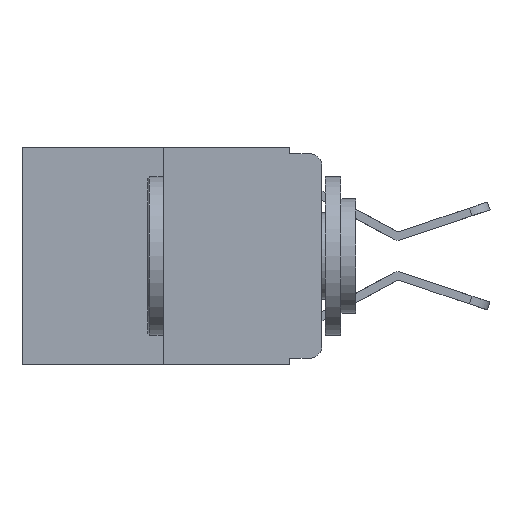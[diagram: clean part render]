
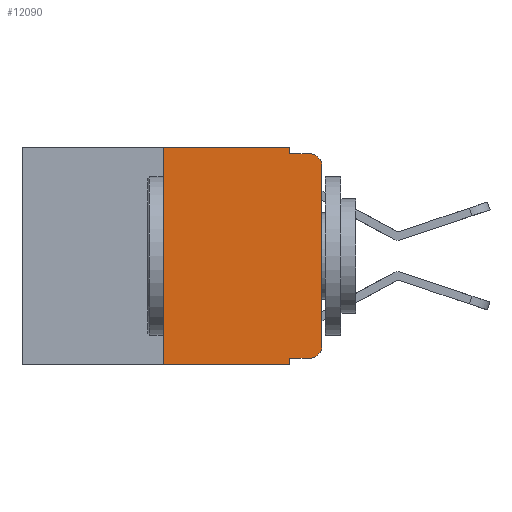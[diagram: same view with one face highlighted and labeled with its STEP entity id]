
A CAD part, left-side view. The second image highlights one B-rep face of the part: STEP entity #12090.
In plain terms, the highlighted planar face has unit normal (-1, 0, 0).
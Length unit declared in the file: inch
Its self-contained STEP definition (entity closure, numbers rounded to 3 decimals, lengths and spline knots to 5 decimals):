
#11 = VECTOR ( 'NONE', #6923, 39.37008 ) ;
#379 = LINE ( 'NONE', #5913, #11 ) ;
#500 = VERTEX_POINT ( 'NONE', #4023 ) ;
#547 = CARTESIAN_POINT ( 'NONE',  ( 0., 0.25, -0.343 ) ) ;
#619 = EDGE_CURVE ( 'NONE', #12169, #500, #5837, .T. ) ;
#708 = CARTESIAN_POINT ( 'NONE',  ( 0., 0.473, -0.343 ) ) ;
#769 = VECTOR ( 'NONE', #8160, 39.37008 ) ;
#1096 = ORIENTED_EDGE ( 'NONE', *, *, #5232, .T. ) ;
#1270 = VECTOR ( 'NONE', #1719, 39.37008 ) ;
#1434 = CARTESIAN_POINT ( 'NONE',  ( 0., 0.051, -0.343 ) ) ;
#1558 = AXIS2_PLACEMENT_3D ( 'NONE', #4679, #11574, #5676 ) ;
#1619 = LINE ( 'NONE', #3967, #1270 ) ;
#1627 = DIRECTION ( 'NONE',  ( 0., 0., -1. ) ) ;
#1719 = DIRECTION ( 'NONE',  ( 0., 0., 1. ) ) ;
#1965 = VERTEX_POINT ( 'NONE', #9014 ) ;
#2000 = ORIENTED_EDGE ( 'NONE', *, *, #619, .F. ) ;
#2155 = AXIS2_PLACEMENT_3D ( 'NONE', #3371, #3324, #12290 ) ;
#2701 = ORIENTED_EDGE ( 'NONE', *, *, #8767, .T. ) ;
#2798 = VECTOR ( 'NONE', #7585, 39.37008 ) ;
#2803 = VERTEX_POINT ( 'NONE', #3824 ) ;
#3264 = EDGE_LOOP ( 'NONE', ( #10030, #10320, #11503, #3905, #2000, #12675, #2701, #10756, #1096, #9434 ) ) ;
#3324 = DIRECTION ( 'NONE',  ( 1., 0., 0. ) ) ;
#3371 = CARTESIAN_POINT ( 'NONE',  ( 0., 0.473, 0. ) ) ;
#3824 = CARTESIAN_POINT ( 'NONE',  ( 0., 0.051, -0.01 ) ) ;
#3861 = EDGE_CURVE ( 'NONE', #9322, #11887, #9301, .T. ) ;
#3905 = ORIENTED_EDGE ( 'NONE', *, *, #7930, .F. ) ;
#3967 = CARTESIAN_POINT ( 'NONE',  ( 0., 0., 0. ) ) ;
#4023 = CARTESIAN_POINT ( 'NONE',  ( 0., 0.051, 0. ) ) ;
#4426 = DIRECTION ( 'NONE',  ( 0., 0., 1. ) ) ;
#4561 = DIRECTION ( 'NONE',  ( 0., -1., 0. ) ) ;
#4667 = CARTESIAN_POINT ( 'NONE',  ( 0., 0.051, -0.333 ) ) ;
#4679 = CARTESIAN_POINT ( 'NONE',  ( 0., 0.02, -0.03 ) ) ;
#5080 = CARTESIAN_POINT ( 'NONE',  ( 0., 0., -0.313 ) ) ;
#5232 = EDGE_CURVE ( 'NONE', #1965, #9322, #8145, .T. ) ;
#5574 = LINE ( 'NONE', #10499, #2798 ) ;
#5676 = DIRECTION ( 'NONE',  ( 0., 0., -1. ) ) ;
#5837 = LINE ( 'NONE', #6064, #10786 ) ;
#5873 = CARTESIAN_POINT ( 'NONE',  ( 0., 0.051, 0. ) ) ;
#5888 = EDGE_CURVE ( 'NONE', #1965, #7457, #10716, .T. ) ;
#5913 = CARTESIAN_POINT ( 'NONE',  ( 0., 0.051, -0.01 ) ) ;
#6064 = CARTESIAN_POINT ( 'NONE',  ( 0., 0.473, 0. ) ) ;
#6923 = DIRECTION ( 'NONE',  ( 0., -1., 0. ) ) ;
#6982 = VERTEX_POINT ( 'NONE', #547 ) ;
#7156 = LINE ( 'NONE', #10394, #12323 ) ;
#7219 = CARTESIAN_POINT ( 'NONE',  ( 0., 0., -0.03 ) ) ;
#7250 = EDGE_CURVE ( 'NONE', #6982, #12169, #7156, .T. ) ;
#7457 = VERTEX_POINT ( 'NONE', #1434 ) ;
#7585 = DIRECTION ( 'NONE',  ( 0., 0., -1. ) ) ;
#7930 = EDGE_CURVE ( 'NONE', #500, #2803, #5574, .T. ) ;
#8145 = LINE ( 'NONE', #4667, #13220 ) ;
#8150 = VECTOR ( 'NONE', #1627, 39.37008 ) ;
#8160 = DIRECTION ( 'NONE',  ( 0., -1., 0. ) ) ;
#8767 = EDGE_CURVE ( 'NONE', #6982, #7457, #11999, .T. ) ;
#9014 = CARTESIAN_POINT ( 'NONE',  ( 0., 0.051, -0.333 ) ) ;
#9268 = EDGE_CURVE ( 'NONE', #2803, #11453, #379, .T. ) ;
#9301 = CIRCLE ( 'NONE', #9639, 0.02 ) ;
#9322 = VERTEX_POINT ( 'NONE', #10923 ) ;
#9434 = ORIENTED_EDGE ( 'NONE', *, *, #3861, .T. ) ;
#9639 = AXIS2_PLACEMENT_3D ( 'NONE', #9780, #10190, #10152 ) ;
#9780 = CARTESIAN_POINT ( 'NONE',  ( 0., 0.02, -0.313 ) ) ;
#9903 = CIRCLE ( 'NONE', #1558, 0.02 ) ;
#10030 = ORIENTED_EDGE ( 'NONE', *, *, #11810, .T. ) ;
#10152 = DIRECTION ( 'NONE',  ( 0., 0., -1. ) ) ;
#10190 = DIRECTION ( 'NONE',  ( -1., 0., 0. ) ) ;
#10320 = ORIENTED_EDGE ( 'NONE', *, *, #10549, .T. ) ;
#10394 = CARTESIAN_POINT ( 'NONE',  ( 0., 0.25, 0. ) ) ;
#10499 = CARTESIAN_POINT ( 'NONE',  ( 0., 0.051, 0. ) ) ;
#10549 = EDGE_CURVE ( 'NONE', #10863, #11453, #9903, .T. ) ;
#10716 = LINE ( 'NONE', #5873, #8150 ) ;
#10756 = ORIENTED_EDGE ( 'NONE', *, *, #5888, .F. ) ;
#10786 = VECTOR ( 'NONE', #11528, 39.37008 ) ;
#10863 = VERTEX_POINT ( 'NONE', #7219 ) ;
#10923 = CARTESIAN_POINT ( 'NONE',  ( 0., 0.02, -0.333 ) ) ;
#11337 = PLANE ( 'NONE',  #2155 ) ;
#11453 = VERTEX_POINT ( 'NONE', #13155 ) ;
#11503 = ORIENTED_EDGE ( 'NONE', *, *, #9268, .F. ) ;
#11528 = DIRECTION ( 'NONE',  ( 0., -1., 0. ) ) ;
#11574 = DIRECTION ( 'NONE',  ( -1., 0., 0. ) ) ;
#11810 = EDGE_CURVE ( 'NONE', #11887, #10863, #1619, .T. ) ;
#11814 = CARTESIAN_POINT ( 'NONE',  ( 0., 0.25, 0. ) ) ;
#11887 = VERTEX_POINT ( 'NONE', #5080 ) ;
#11999 = LINE ( 'NONE', #708, #769 ) ;
#12090 = ADVANCED_FACE ( 'NONE', ( #13248 ), #11337, .F. ) ;
#12169 = VERTEX_POINT ( 'NONE', #11814 ) ;
#12290 = DIRECTION ( 'NONE',  ( 0., 0., -1. ) ) ;
#12323 = VECTOR ( 'NONE', #4426, 39.37008 ) ;
#12675 = ORIENTED_EDGE ( 'NONE', *, *, #7250, .F. ) ;
#13155 = CARTESIAN_POINT ( 'NONE',  ( 0., 0.02, -0.01 ) ) ;
#13220 = VECTOR ( 'NONE', #4561, 39.37008 ) ;
#13248 = FACE_OUTER_BOUND ( 'NONE', #3264, .T. ) ;
